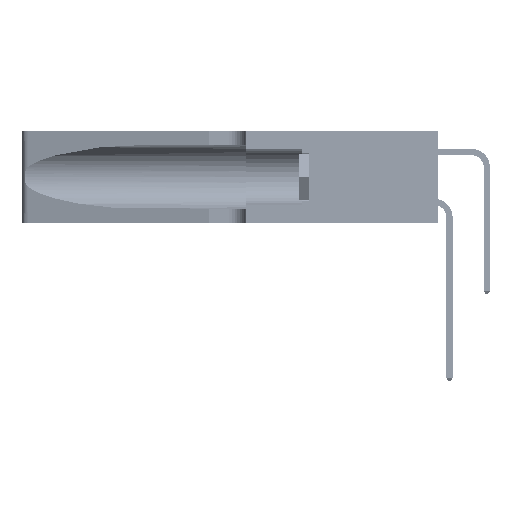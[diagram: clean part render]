
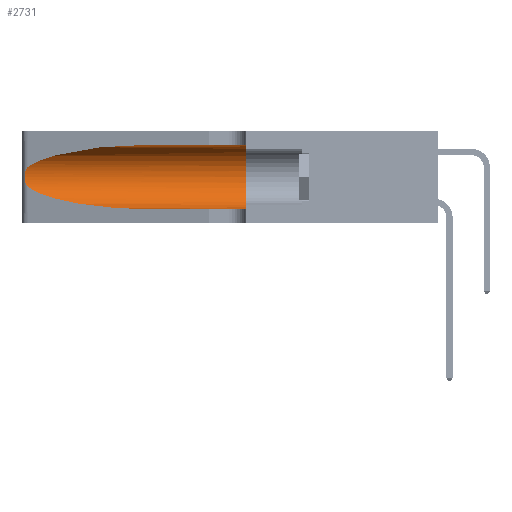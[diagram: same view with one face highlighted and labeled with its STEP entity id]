
A CAD part, left-side view. The second image highlights one B-rep face of the part: STEP entity #2731.
In plain terms, the highlighted cylindrical face has radius 3.308 mm (diameter 6.617 mm), a partial arc.
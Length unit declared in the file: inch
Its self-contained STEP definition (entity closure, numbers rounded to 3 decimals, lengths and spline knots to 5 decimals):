
#2430 = CARTESIAN_POINT ( 'NONE',  ( 0.25787, 1.23484, 0.2124 ) ) ;
#2731 = ADVANCED_FACE ( 'NONE', ( #23716 ), #12691, .F. ) ;
#6265 = CARTESIAN_POINT ( 'NONE',  ( 0.26075, 1.23896, 0.178 ) ) ;
#6798 = CARTESIAN_POINT ( 'NONE',  ( 0.26017, 1.23833, 0.17102 ) ) ;
#6969 = B_SPLINE_CURVE_WITH_KNOTS ( 'NONE', 3,
 ( #48029, #23116, #52038, #2430, #27264, #35461, #26750, #6265, #6798, #27098, #10603, #14577, #31459, #35280 ),
 .UNSPECIFIED., .F., .F.,
 ( 4, 2, 2, 2, 2, 2, 4 ),
 ( 0., 0.00027, 0.00053, 0.00107, 0.0016, 0.00187, 0.00214 ),
 .UNSPECIFIED. ) ;
#9186 = ORIENTED_EDGE ( 'NONE', *, *, #42208, .T. ) ;
#10213 = ORIENTED_EDGE ( 'NONE', *, *, #45057, .F. ) ;
#10278 = VERTEX_POINT ( 'NONE', #26925 ) ;
#10603 = CARTESIAN_POINT ( 'NONE',  ( 0.25789, 1.23486, 0.15765 ) ) ;
#11021 = CARTESIAN_POINT ( 'NONE',  ( 0.1305, 0.35, 0.31525 ) ) ;
#11347 = CARTESIAN_POINT ( 'NONE',  ( 0.25487, 1.22718, 0.22369 ) ) ;
#12691 = CYLINDRICAL_SURFACE ( 'NONE', #18608, 0.13025 ) ;
#14577 = CARTESIAN_POINT ( 'NONE',  ( 0.25639, 1.23186, 0.15144 ) ) ;
#14889 = CARTESIAN_POINT ( 'NONE',  ( 0.1305, 1.61858, 0.185 ) ) ;
#15370 = LINE ( 'NONE', #27834, #25736 ) ;
#16022 = VERTEX_POINT ( 'NONE', #44370 ) ;
#16816 = VECTOR ( 'NONE', #49365, 39.37008 ) ;
#18592 =( BOUNDED_CURVE ( )  B_SPLINE_CURVE ( 3, ( #47846, #18614, #22596, #22765 ),
 .UNSPECIFIED., .F., .T. ) 
 B_SPLINE_CURVE_WITH_KNOTS ( ( 4, 4 ),
 ( 3.44316, 4.71239 ),
 .UNSPECIFIED. ) 
 CURVE ( )  GEOMETRIC_REPRESENTATION_ITEM ( )  RATIONAL_B_SPLINE_CURVE ( ( 1., 0.87, 0.87, 1. ) ) 
 REPRESENTATION_ITEM ( '' )  );
#18608 = AXIS2_PLACEMENT_3D ( 'NONE', #14889, #31062, #18743 ) ;
#18614 = CARTESIAN_POINT ( 'NONE',  ( 0.2373, 1.15595, 0.08982 ) ) ;
#18743 = DIRECTION ( 'NONE',  ( 0., 0., -1. ) ) ;
#19580 = CARTESIAN_POINT ( 'NONE',  ( 0.2373, 1.15595, 0.28018 ) ) ;
#22188 = DIRECTION ( 'NONE',  ( 0., 0., 1. ) ) ;
#22367 = ORIENTED_EDGE ( 'NONE', *, *, #22773, .T. ) ;
#22596 = CARTESIAN_POINT ( 'NONE',  ( 0.18966, 0.96281, 0.05475 ) ) ;
#22609 = CARTESIAN_POINT ( 'NONE',  ( 0.1305, 0.35, 0.05475 ) ) ;
#22762 = VERTEX_POINT ( 'NONE', #51331 ) ;
#22765 = CARTESIAN_POINT ( 'NONE',  ( 0.1305, 0.72297, 0.05475 ) ) ;
#22773 = EDGE_CURVE ( 'NONE', #26775, #16022, #6969, .T. ) ;
#23116 = CARTESIAN_POINT ( 'NONE',  ( 0.25555, 1.22994, 0.2215 ) ) ;
#23567 = CARTESIAN_POINT ( 'NONE',  ( 0.1305, 0.72297, 0.31525 ) ) ;
#23716 = FACE_OUTER_BOUND ( 'NONE', #24390, .T. ) ;
#24293 = AXIS2_PLACEMENT_3D ( 'NONE', #47259, #47077, #22188 ) ;
#24390 = EDGE_LOOP ( 'NONE', ( #47884, #22367, #9186, #41392, #47224, #10213 ) ) ;
#24604 = VERTEX_POINT ( 'NONE', #22609 ) ;
#25230 = EDGE_CURVE ( 'NONE', #44837, #24604, #36015, .T. ) ;
#25736 = VECTOR ( 'NONE', #32021, 39.37008 ) ;
#26051 = EDGE_CURVE ( 'NONE', #10278, #26775, #27882, .T. ) ;
#26750 = CARTESIAN_POINT ( 'NONE',  ( 0.26075, 1.23896, 0.19203 ) ) ;
#26775 = VERTEX_POINT ( 'NONE', #11347 ) ;
#26925 = CARTESIAN_POINT ( 'NONE',  ( 0.1305, 0.72297, 0.31525 ) ) ;
#27098 = CARTESIAN_POINT ( 'NONE',  ( 0.25856, 1.23593, 0.16098 ) ) ;
#27264 = CARTESIAN_POINT ( 'NONE',  ( 0.25854, 1.2359, 0.20912 ) ) ;
#27724 = CARTESIAN_POINT ( 'NONE',  ( 0.18966, 0.96281, 0.31525 ) ) ;
#27834 = CARTESIAN_POINT ( 'NONE',  ( 0.1305, 1.61858, 0.05475 ) ) ;
#27882 =( BOUNDED_CURVE ( )  B_SPLINE_CURVE ( 3, ( #23567, #27724, #19580, #44093 ),
 .UNSPECIFIED., .F., .F. ) 
 B_SPLINE_CURVE_WITH_KNOTS ( ( 4, 4 ),
 ( 1.5708, 2.84003 ),
 .UNSPECIFIED. ) 
 CURVE ( )  GEOMETRIC_REPRESENTATION_ITEM ( )  RATIONAL_B_SPLINE_CURVE ( ( 1., 0.87, 0.87, 1. ) ) 
 REPRESENTATION_ITEM ( '' )  );
#31062 = DIRECTION ( 'NONE',  ( 0., -1., 0. ) ) ;
#31459 = CARTESIAN_POINT ( 'NONE',  ( 0.25555, 1.22993, 0.14849 ) ) ;
#32021 = DIRECTION ( 'NONE',  ( 0., -1., 0. ) ) ;
#35280 = CARTESIAN_POINT ( 'NONE',  ( 0.25487, 1.22718, 0.14631 ) ) ;
#35461 = CARTESIAN_POINT ( 'NONE',  ( 0.26018, 1.23835, 0.19895 ) ) ;
#36015 = CIRCLE ( 'NONE', #24293, 0.13025 ) ;
#36823 = CARTESIAN_POINT ( 'NONE',  ( 0.1305, 1.61858, 0.31525 ) ) ;
#41392 = ORIENTED_EDGE ( 'NONE', *, *, #52561, .T. ) ;
#42208 = EDGE_CURVE ( 'NONE', #16022, #22762, #18592, .T. ) ;
#44093 = CARTESIAN_POINT ( 'NONE',  ( 0.25487, 1.22718, 0.22369 ) ) ;
#44370 = CARTESIAN_POINT ( 'NONE',  ( 0.25487, 1.22718, 0.14631 ) ) ;
#44837 = VERTEX_POINT ( 'NONE', #11021 ) ;
#45057 = EDGE_CURVE ( 'NONE', #10278, #44837, #53202, .T. ) ;
#47077 = DIRECTION ( 'NONE',  ( 0., 1., 0. ) ) ;
#47224 = ORIENTED_EDGE ( 'NONE', *, *, #25230, .F. ) ;
#47259 = CARTESIAN_POINT ( 'NONE',  ( 0.1305, 0.35, 0.185 ) ) ;
#47846 = CARTESIAN_POINT ( 'NONE',  ( 0.25487, 1.22718, 0.14631 ) ) ;
#47884 = ORIENTED_EDGE ( 'NONE', *, *, #26051, .T. ) ;
#48029 = CARTESIAN_POINT ( 'NONE',  ( 0.25487, 1.22718, 0.22369 ) ) ;
#49365 = DIRECTION ( 'NONE',  ( 0., -1., 0. ) ) ;
#51331 = CARTESIAN_POINT ( 'NONE',  ( 0.1305, 0.72297, 0.05475 ) ) ;
#52038 = CARTESIAN_POINT ( 'NONE',  ( 0.25639, 1.23184, 0.21858 ) ) ;
#52561 = EDGE_CURVE ( 'NONE', #22762, #24604, #15370, .T. ) ;
#53202 = LINE ( 'NONE', #36823, #16816 ) ;
